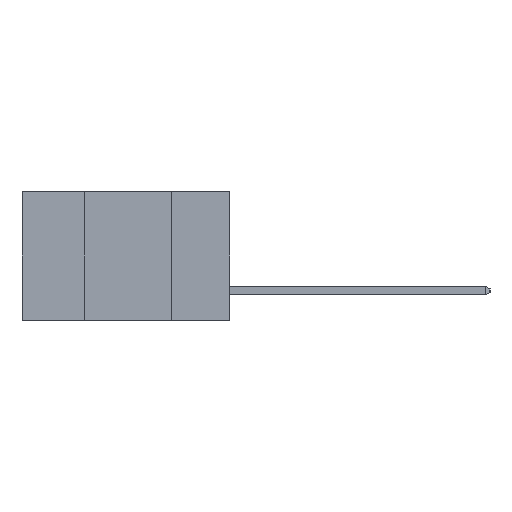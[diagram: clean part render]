
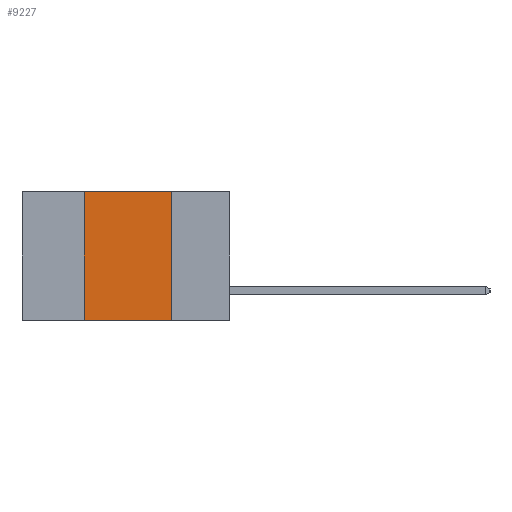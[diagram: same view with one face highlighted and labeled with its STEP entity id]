
A CAD part, left-side view. The second image highlights one B-rep face of the part: STEP entity #9227.
In plain terms, the highlighted planar face has unit normal (-1, 0, 0).
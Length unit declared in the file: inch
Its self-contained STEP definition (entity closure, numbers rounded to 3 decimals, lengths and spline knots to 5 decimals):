
#1581 = ORIENTED_EDGE ( 'NONE', *, *, #5929, .F. ) ;
#2104 = DIRECTION ( 'NONE',  ( 0., 0., -1. ) ) ;
#2161 = DIRECTION ( 'NONE',  ( 0., -1., 0. ) ) ;
#3476 = PLANE ( 'NONE',  #6246 ) ;
#3488 = LINE ( 'NONE', #10592, #8664 ) ;
#3665 = EDGE_CURVE ( 'NONE', #4166, #8191, #10338, .T. ) ;
#3855 = EDGE_CURVE ( 'NONE', #3984, #6819, #10183, .T. ) ;
#3984 = VERTEX_POINT ( 'NONE', #4163 ) ;
#4163 = CARTESIAN_POINT ( 'NONE',  ( 0., 0.17, 0. ) ) ;
#4166 = VERTEX_POINT ( 'NONE', #12697 ) ;
#4515 = DIRECTION ( 'NONE',  ( 0., -1., 0. ) ) ;
#4557 = CARTESIAN_POINT ( 'NONE',  ( 0., 0.6, 0. ) ) ;
#5566 = DIRECTION ( 'NONE',  ( 1., 0., 0. ) ) ;
#5929 = EDGE_CURVE ( 'NONE', #8191, #3984, #8078, .T. ) ;
#6246 = AXIS2_PLACEMENT_3D ( 'NONE', #4557, #5566, #12595 ) ;
#6819 = VERTEX_POINT ( 'NONE', #7623 ) ;
#7623 = CARTESIAN_POINT ( 'NONE',  ( 0., 0.17, -0.37 ) ) ;
#7850 = CARTESIAN_POINT ( 'NONE',  ( 0., 0.42, 0. ) ) ;
#8019 = ORIENTED_EDGE ( 'NONE', *, *, #3665, .F. ) ;
#8078 = LINE ( 'NONE', #13288, #13003 ) ;
#8191 = VERTEX_POINT ( 'NONE', #7850 ) ;
#8664 = VECTOR ( 'NONE', #4515, 39.37008 ) ;
#8695 = EDGE_CURVE ( 'NONE', #4166, #6819, #3488, .T. ) ;
#9163 = ORIENTED_EDGE ( 'NONE', *, *, #8695, .T. ) ;
#9227 = ADVANCED_FACE ( 'NONE', ( #12935 ), #3476, .F. ) ;
#9364 = DIRECTION ( 'NONE',  ( 0., 0., 1. ) ) ;
#10183 = LINE ( 'NONE', #10610, #12776 ) ;
#10218 = CARTESIAN_POINT ( 'NONE',  ( 0., 0.42, -0.37 ) ) ;
#10338 = LINE ( 'NONE', #10218, #12633 ) ;
#10592 = CARTESIAN_POINT ( 'NONE',  ( 0., 0.6, -0.37 ) ) ;
#10610 = CARTESIAN_POINT ( 'NONE',  ( 0., 0.17, -0.37 ) ) ;
#11889 = ORIENTED_EDGE ( 'NONE', *, *, #3855, .F. ) ;
#12580 = EDGE_LOOP ( 'NONE', ( #11889, #1581, #8019, #9163 ) ) ;
#12595 = DIRECTION ( 'NONE',  ( 0., 0., -1. ) ) ;
#12633 = VECTOR ( 'NONE', #9364, 39.37008 ) ;
#12697 = CARTESIAN_POINT ( 'NONE',  ( 0., 0.42, -0.37 ) ) ;
#12776 = VECTOR ( 'NONE', #2104, 39.37008 ) ;
#12935 = FACE_OUTER_BOUND ( 'NONE', #12580, .T. ) ;
#13003 = VECTOR ( 'NONE', #2161, 39.37008 ) ;
#13288 = CARTESIAN_POINT ( 'NONE',  ( 0., 0.6, 0. ) ) ;
